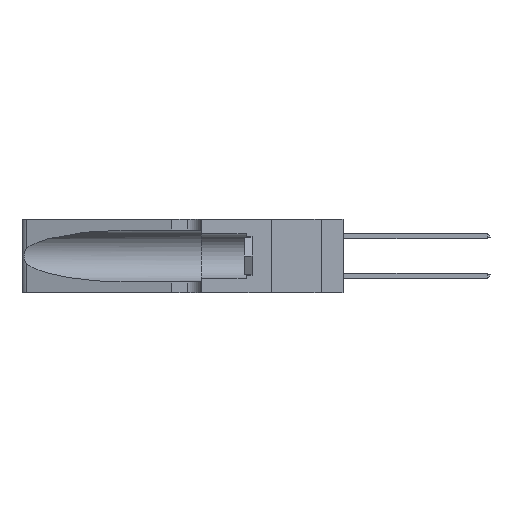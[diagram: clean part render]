
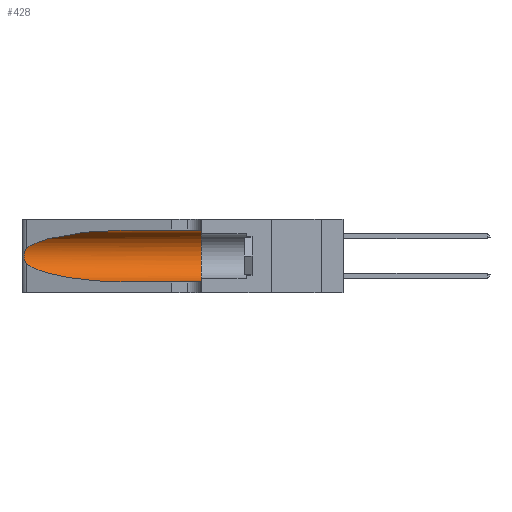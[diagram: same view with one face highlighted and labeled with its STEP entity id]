
A CAD part, left-side view. The second image highlights one B-rep face of the part: STEP entity #428.
In plain terms, the highlighted cylindrical face has radius 3.308 mm (diameter 6.617 mm), a partial arc.
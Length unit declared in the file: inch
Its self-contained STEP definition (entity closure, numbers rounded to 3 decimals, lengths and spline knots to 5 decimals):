
#207 = CARTESIAN_POINT ( 'NONE',  ( 0.1305, 0.72297, 0.05475 ) ) ;
#224 = ORIENTED_EDGE ( 'NONE', *, *, #18931, .T. ) ;
#347 = DIRECTION ( 'NONE',  ( 0., -1., 0. ) ) ;
#428 = ADVANCED_FACE ( 'NONE', ( #26125 ), #7086, .F. ) ;
#1525 = AXIS2_PLACEMENT_3D ( 'NONE', #4614, #5367, #5159 ) ;
#2024 = CARTESIAN_POINT ( 'NONE',  ( 0.26018, 1.23835, 0.19895 ) ) ;
#2630 = CARTESIAN_POINT ( 'NONE',  ( 0.1305, 0.35, 0.31525 ) ) ;
#3000 = VERTEX_POINT ( 'NONE', #207 ) ;
#3694 = EDGE_LOOP ( 'NONE', ( #24773, #8233, #21307, #224, #19312, #28499 ) ) ;
#4408 = CARTESIAN_POINT ( 'NONE',  ( 0.25555, 1.22994, 0.2215 ) ) ;
#4524 = CARTESIAN_POINT ( 'NONE',  ( 0.26075, 1.23896, 0.178 ) ) ;
#4608 = DIRECTION ( 'NONE',  ( 0., 1., 0. ) ) ;
#4614 = CARTESIAN_POINT ( 'NONE',  ( 0.1305, 1.61858, 0.185 ) ) ;
#5159 = DIRECTION ( 'NONE',  ( 0., 0., -1. ) ) ;
#5367 = DIRECTION ( 'NONE',  ( 0., -1., 0. ) ) ;
#5427 = VERTEX_POINT ( 'NONE', #24362 ) ;
#6071 = LINE ( 'NONE', #22230, #12580 ) ;
#6820 = CARTESIAN_POINT ( 'NONE',  ( 0.25487, 1.22718, 0.14631 ) ) ;
#7086 = CYLINDRICAL_SURFACE ( 'NONE', #1525, 0.13025 ) ;
#7094 = CARTESIAN_POINT ( 'NONE',  ( 0.25856, 1.23593, 0.16098 ) ) ;
#7399 =( BOUNDED_CURVE ( )  B_SPLINE_CURVE ( 3, ( #13456, #20575, #13544, #30041 ),
 .UNSPECIFIED., .F., .F. ) 
 B_SPLINE_CURVE_WITH_KNOTS ( ( 4, 4 ),
 ( 1.5708, 2.84003 ),
 .UNSPECIFIED. ) 
 CURVE ( )  GEOMETRIC_REPRESENTATION_ITEM ( )  RATIONAL_B_SPLINE_CURVE ( ( 1., 0.87, 0.87, 1. ) ) 
 REPRESENTATION_ITEM ( '' )  );
#7924 = LINE ( 'NONE', #24851, #14357 ) ;
#8174 = DIRECTION ( 'NONE',  ( 0., -1., 0. ) ) ;
#8233 = ORIENTED_EDGE ( 'NONE', *, *, #21462, .T. ) ;
#8391 =( BOUNDED_CURVE ( )  B_SPLINE_CURVE ( 3, ( #6820, #21176, #23543, #9283 ),
 .UNSPECIFIED., .F., .F. ) 
 B_SPLINE_CURVE_WITH_KNOTS ( ( 4, 4 ),
 ( 3.44316, 4.71239 ),
 .UNSPECIFIED. ) 
 CURVE ( )  GEOMETRIC_REPRESENTATION_ITEM ( )  RATIONAL_B_SPLINE_CURVE ( ( 1., 0.87, 0.87, 1. ) ) 
 REPRESENTATION_ITEM ( '' )  );
#9283 = CARTESIAN_POINT ( 'NONE',  ( 0.1305, 0.72297, 0.05475 ) ) ;
#9558 = CARTESIAN_POINT ( 'NONE',  ( 0.25639, 1.23186, 0.15144 ) ) ;
#9813 = EDGE_CURVE ( 'NONE', #5427, #29351, #7399, .T. ) ;
#11969 = CARTESIAN_POINT ( 'NONE',  ( 0.25487, 1.22718, 0.14631 ) ) ;
#12580 = VECTOR ( 'NONE', #347, 39.37008 ) ;
#13456 = CARTESIAN_POINT ( 'NONE',  ( 0.1305, 0.72297, 0.31525 ) ) ;
#13533 = CARTESIAN_POINT ( 'NONE',  ( 0.1305, 0.35, 0.05475 ) ) ;
#13544 = CARTESIAN_POINT ( 'NONE',  ( 0.2373, 1.15595, 0.28018 ) ) ;
#14307 = CARTESIAN_POINT ( 'NONE',  ( 0.25639, 1.23184, 0.21858 ) ) ;
#14357 = VECTOR ( 'NONE', #8174, 39.37008 ) ;
#15608 = VERTEX_POINT ( 'NONE', #13533 ) ;
#16066 = VERTEX_POINT ( 'NONE', #21295 ) ;
#16703 = CARTESIAN_POINT ( 'NONE',  ( 0.25854, 1.2359, 0.20912 ) ) ;
#17575 = CIRCLE ( 'NONE', #18423, 0.13025 ) ;
#18423 = AXIS2_PLACEMENT_3D ( 'NONE', #19129, #4608, #21510 ) ;
#18931 = EDGE_CURVE ( 'NONE', #3000, #15608, #7924, .T. ) ;
#19064 = CARTESIAN_POINT ( 'NONE',  ( 0.26075, 1.23896, 0.19203 ) ) ;
#19129 = CARTESIAN_POINT ( 'NONE',  ( 0.1305, 0.35, 0.185 ) ) ;
#19312 = ORIENTED_EDGE ( 'NONE', *, *, #28315, .F. ) ;
#20575 = CARTESIAN_POINT ( 'NONE',  ( 0.18966, 0.96281, 0.31525 ) ) ;
#21176 = CARTESIAN_POINT ( 'NONE',  ( 0.2373, 1.15595, 0.08982 ) ) ;
#21295 = CARTESIAN_POINT ( 'NONE',  ( 0.25487, 1.22718, 0.14631 ) ) ;
#21307 = ORIENTED_EDGE ( 'NONE', *, *, #30740, .T. ) ;
#21436 = CARTESIAN_POINT ( 'NONE',  ( 0.26017, 1.23833, 0.17102 ) ) ;
#21462 = EDGE_CURVE ( 'NONE', #29351, #16066, #30464, .T. ) ;
#21510 = DIRECTION ( 'NONE',  ( 0., 0., 1. ) ) ;
#22230 = CARTESIAN_POINT ( 'NONE',  ( 0.1305, 1.61858, 0.31525 ) ) ;
#23543 = CARTESIAN_POINT ( 'NONE',  ( 0.18966, 0.96281, 0.05475 ) ) ;
#23808 = CARTESIAN_POINT ( 'NONE',  ( 0.25789, 1.23486, 0.15765 ) ) ;
#24310 = EDGE_CURVE ( 'NONE', #5427, #28480, #6071, .T. ) ;
#24362 = CARTESIAN_POINT ( 'NONE',  ( 0.1305, 0.72297, 0.31525 ) ) ;
#24773 = ORIENTED_EDGE ( 'NONE', *, *, #9813, .T. ) ;
#24851 = CARTESIAN_POINT ( 'NONE',  ( 0.1305, 1.61858, 0.05475 ) ) ;
#26125 = FACE_OUTER_BOUND ( 'NONE', #3694, .T. ) ;
#26170 = CARTESIAN_POINT ( 'NONE',  ( 0.25555, 1.22993, 0.14849 ) ) ;
#27528 = CARTESIAN_POINT ( 'NONE',  ( 0.25487, 1.22718, 0.22369 ) ) ;
#28315 = EDGE_CURVE ( 'NONE', #28480, #15608, #17575, .T. ) ;
#28480 = VERTEX_POINT ( 'NONE', #2630 ) ;
#28499 = ORIENTED_EDGE ( 'NONE', *, *, #24310, .F. ) ;
#29351 = VERTEX_POINT ( 'NONE', #27528 ) ;
#30041 = CARTESIAN_POINT ( 'NONE',  ( 0.25487, 1.22718, 0.22369 ) ) ;
#30464 = B_SPLINE_CURVE_WITH_KNOTS ( 'NONE', 3,
 ( #30694, #4408, #14307, #30796, #16703, #2024, #19064, #4524, #21436, #7094, #23808, #9558, #26170, #11969 ),
 .UNSPECIFIED., .F., .F.,
 ( 4, 2, 2, 2, 2, 2, 4 ),
 ( 0., 0.00027, 0.00053, 0.00107, 0.0016, 0.00187, 0.00214 ),
 .UNSPECIFIED. ) ;
#30694 = CARTESIAN_POINT ( 'NONE',  ( 0.25487, 1.22718, 0.22369 ) ) ;
#30740 = EDGE_CURVE ( 'NONE', #16066, #3000, #8391, .T. ) ;
#30796 = CARTESIAN_POINT ( 'NONE',  ( 0.25787, 1.23484, 0.2124 ) ) ;
